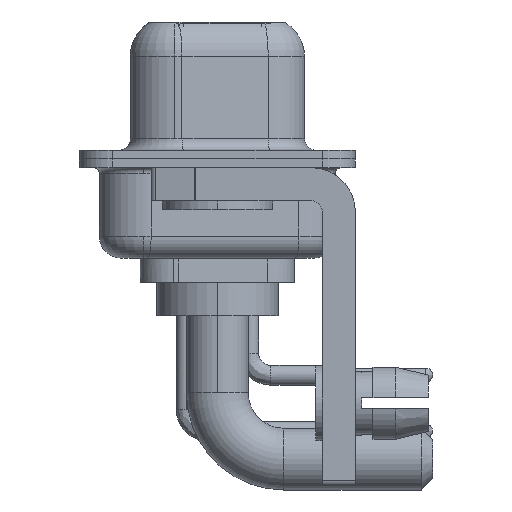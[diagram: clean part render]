
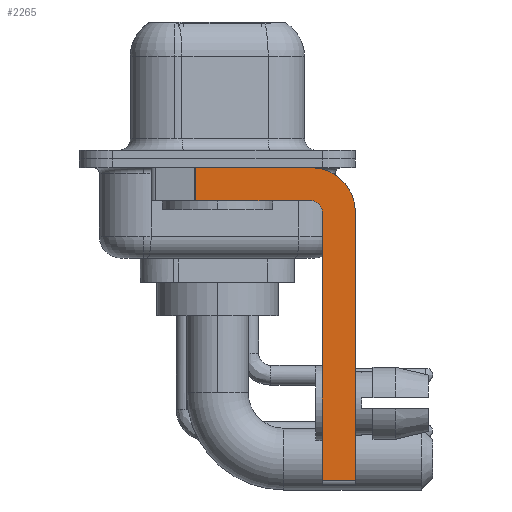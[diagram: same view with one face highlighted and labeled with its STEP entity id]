
A CAD part, left-side view. The second image highlights one B-rep face of the part: STEP entity #2265.
In plain terms, the highlighted planar face has unit normal (-1, 0, 0).
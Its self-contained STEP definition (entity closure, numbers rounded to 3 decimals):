
#263 = LINE ( 'NONE', #3146, #14359 ) ;
#491 = ORIENTED_EDGE ( 'NONE', *, *, #7153, .F. ) ;
#504 = CARTESIAN_POINT ( 'NONE',  ( -2.9, -4.25, -2.4 ) ) ;
#790 = EDGE_CURVE ( 'NONE', #16878, #16044, #15962, .T. ) ;
#1037 = VECTOR ( 'NONE', #16522, 1000. ) ;
#2169 = CARTESIAN_POINT ( 'NONE',  ( -2.9, -4.25, -0.4 ) ) ;
#2265 = ADVANCED_FACE ( 'NONE', ( #9377 ), #9569, .F. ) ;
#2281 = CARTESIAN_POINT ( 'NONE',  ( -2.9, -4.25, -2.4 ) ) ;
#2664 = CARTESIAN_POINT ( 'NONE',  ( -2.9, 3., -0.4 ) ) ;
#2687 = LINE ( 'NONE', #11554, #14171 ) ;
#2856 = ORIENTED_EDGE ( 'NONE', *, *, #790, .F. ) ;
#2929 = VECTOR ( 'NONE', #19375, 1000. ) ;
#3119 = VERTEX_POINT ( 'NONE', #7685 ) ;
#3146 = CARTESIAN_POINT ( 'NONE',  ( -2.9, -4.25, -14.55 ) ) ;
#3516 = EDGE_CURVE ( 'NONE', #17849, #9438, #13166, .T. ) ;
#3567 = AXIS2_PLACEMENT_3D ( 'NONE', #13545, #19591, #12048 ) ;
#3917 = AXIS2_PLACEMENT_3D ( 'NONE', #504, #18520, #12450 ) ;
#4260 = LINE ( 'NONE', #2664, #2929 ) ;
#4546 = DIRECTION ( 'NONE',  ( 0., 0., -1. ) ) ;
#4884 = ORIENTED_EDGE ( 'NONE', *, *, #10776, .F. ) ;
#5341 = DIRECTION ( 'NONE',  ( -1., 0., 0. ) ) ;
#5725 = CARTESIAN_POINT ( 'NONE',  ( -2.9, 0.978, -1.9 ) ) ;
#5763 = VECTOR ( 'NONE', #4546, 1000. ) ;
#6548 = CARTESIAN_POINT ( 'NONE',  ( -2.9, -6.25, -2.4 ) ) ;
#6723 = CARTESIAN_POINT ( 'NONE',  ( -2.9, -4.75, -14.55 ) ) ;
#6813 = ORIENTED_EDGE ( 'NONE', *, *, #10967, .T. ) ;
#6818 = ORIENTED_EDGE ( 'NONE', *, *, #10628, .T. ) ;
#7153 = EDGE_CURVE ( 'NONE', #16044, #15687, #9252, .T. ) ;
#7349 = AXIS2_PLACEMENT_3D ( 'NONE', #2281, #5341, #14614 ) ;
#7671 = EDGE_LOOP ( 'NONE', ( #16532, #6813, #13455, #4884, #16776, #6818, #491, #2856 ) ) ;
#7685 = CARTESIAN_POINT ( 'NONE',  ( -2.9, 0.978, -1.9 ) ) ;
#8582 = DIRECTION ( 'NONE',  ( 0., 0., 1. ) ) ;
#8660 = DIRECTION ( 'NONE',  ( 0., 1., 0. ) ) ;
#8788 = CARTESIAN_POINT ( 'NONE',  ( -2.9, -6.25, -14.55 ) ) ;
#9252 = LINE ( 'NONE', #13641, #1037 ) ;
#9374 = CARTESIAN_POINT ( 'NONE',  ( -2.9, 0.978, -0.4 ) ) ;
#9377 = FACE_OUTER_BOUND ( 'NONE', #7671, .T. ) ;
#9438 = VERTEX_POINT ( 'NONE', #13616 ) ;
#9569 = PLANE ( 'NONE',  #3917 ) ;
#10628 = EDGE_CURVE ( 'NONE', #17849, #15687, #263, .T. ) ;
#10776 = EDGE_CURVE ( 'NONE', #9438, #14165, #11817, .T. ) ;
#10816 = DIRECTION ( 'NONE',  ( 0., -1., 0. ) ) ;
#10957 = EDGE_CURVE ( 'NONE', #12296, #16878, #4260, .T. ) ;
#10967 = EDGE_CURVE ( 'NONE', #12296, #3119, #16407, .T. ) ;
#11554 = CARTESIAN_POINT ( 'NONE',  ( -2.9, -4.25, -1.9 ) ) ;
#11817 = CIRCLE ( 'NONE', #7349, 0.5 ) ;
#12048 = DIRECTION ( 'NONE',  ( 0., 0., -1. ) ) ;
#12296 = VERTEX_POINT ( 'NONE', #9374 ) ;
#12450 = DIRECTION ( 'NONE',  ( 0., 0., -1. ) ) ;
#13166 = LINE ( 'NONE', #16147, #16644 ) ;
#13455 = ORIENTED_EDGE ( 'NONE', *, *, #16159, .F. ) ;
#13545 = CARTESIAN_POINT ( 'NONE',  ( -2.9, -4.25, -2.4 ) ) ;
#13616 = CARTESIAN_POINT ( 'NONE',  ( -2.9, -4.75, -2.4 ) ) ;
#13641 = CARTESIAN_POINT ( 'NONE',  ( -2.9, -6.25, -2.4 ) ) ;
#14165 = VERTEX_POINT ( 'NONE', #14188 ) ;
#14171 = VECTOR ( 'NONE', #8660, 1000. ) ;
#14188 = CARTESIAN_POINT ( 'NONE',  ( -2.9, -4.25, -1.9 ) ) ;
#14359 = VECTOR ( 'NONE', #10816, 1000. ) ;
#14614 = DIRECTION ( 'NONE',  ( 0., 0., 1. ) ) ;
#15687 = VERTEX_POINT ( 'NONE', #8788 ) ;
#15962 = CIRCLE ( 'NONE', #3567, 2. ) ;
#16044 = VERTEX_POINT ( 'NONE', #6548 ) ;
#16147 = CARTESIAN_POINT ( 'NONE',  ( -2.9, -4.75, -14.8 ) ) ;
#16159 = EDGE_CURVE ( 'NONE', #14165, #3119, #2687, .T. ) ;
#16407 = LINE ( 'NONE', #5725, #5763 ) ;
#16522 = DIRECTION ( 'NONE',  ( 0., 0., -1. ) ) ;
#16532 = ORIENTED_EDGE ( 'NONE', *, *, #10957, .F. ) ;
#16644 = VECTOR ( 'NONE', #8582, 1000. ) ;
#16776 = ORIENTED_EDGE ( 'NONE', *, *, #3516, .F. ) ;
#16878 = VERTEX_POINT ( 'NONE', #2169 ) ;
#17849 = VERTEX_POINT ( 'NONE', #6723 ) ;
#18520 = DIRECTION ( 'NONE',  ( 1., 0., 0. ) ) ;
#19375 = DIRECTION ( 'NONE',  ( 0., -1., 0. ) ) ;
#19591 = DIRECTION ( 'NONE',  ( 1., 0., 0. ) ) ;
